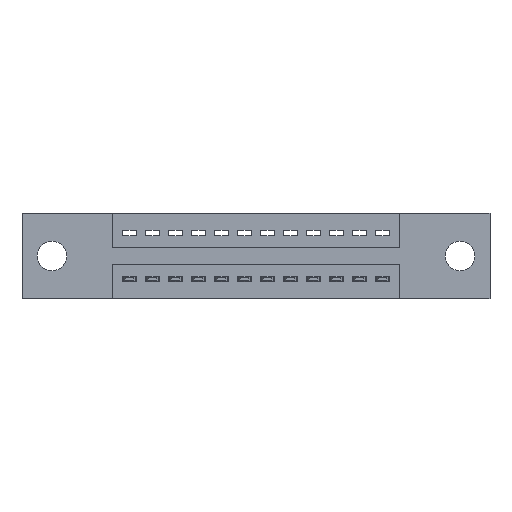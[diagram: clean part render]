
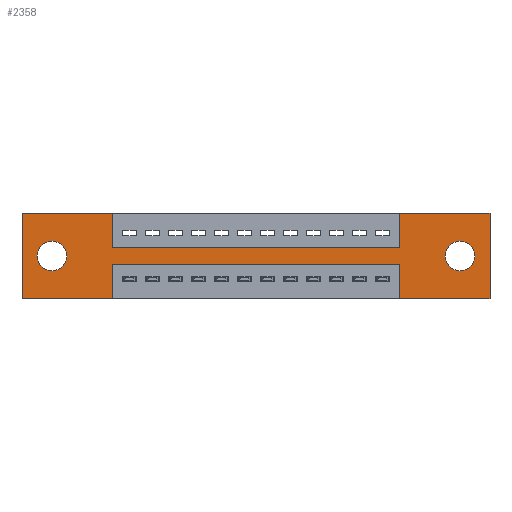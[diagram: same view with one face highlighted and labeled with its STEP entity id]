
A CAD part, front view. The second image highlights one B-rep face of the part: STEP entity #2358.
In plain terms, the highlighted planar face has unit normal (0, -1, 0).
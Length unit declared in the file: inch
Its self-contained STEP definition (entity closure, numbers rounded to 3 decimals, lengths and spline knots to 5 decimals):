
#106 = VECTOR ( 'NONE', #5820, 39.37008 ) ;
#159 = CARTESIAN_POINT ( 'NONE',  ( 2.035, 0., 0. ) ) ;
#206 = LINE ( 'NONE', #3514, #5138 ) ;
#230 = CIRCLE ( 'NONE', #300, 0.064 ) ;
#300 = AXIS2_PLACEMENT_3D ( 'NONE', #12722, #7587, #6706 ) ;
#420 = VERTEX_POINT ( 'NONE', #12027 ) ;
#423 = LINE ( 'NONE', #4810, #106 ) ;
#499 = EDGE_CURVE ( 'NONE', #1969, #12768, #10597, .T. ) ;
#566 = LINE ( 'NONE', #1844, #1185 ) ;
#683 = EDGE_CURVE ( 'NONE', #12281, #10025, #2646, .T. ) ;
#874 = CARTESIAN_POINT ( 'NONE',  ( 0., 0., 0. ) ) ;
#915 = EDGE_LOOP ( 'NONE', ( #11493, #12280, #1550, #6543, #5433, #10860, #11381, #11268, #9116, #10069, #10234, #10438 ) ) ;
#1167 = DIRECTION ( 'NONE',  ( 0., 0., 1. ) ) ;
#1185 = VECTOR ( 'NONE', #2831, 39.37008 ) ;
#1343 = AXIS2_PLACEMENT_3D ( 'NONE', #11222, #5235, #12247 ) ;
#1377 = EDGE_CURVE ( 'NONE', #10025, #3763, #12811, .T. ) ;
#1464 = EDGE_CURVE ( 'NONE', #9595, #420, #11556, .T. ) ;
#1539 = DIRECTION ( 'NONE',  ( 1., 0., 0. ) ) ;
#1550 = ORIENTED_EDGE ( 'NONE', *, *, #7422, .F. ) ;
#1815 = CARTESIAN_POINT ( 'NONE',  ( 1.6425, 0., -0.22 ) ) ;
#1825 = LINE ( 'NONE', #11858, #12153 ) ;
#1844 = CARTESIAN_POINT ( 'NONE',  ( 0., 0., -0.37 ) ) ;
#1969 = VERTEX_POINT ( 'NONE', #10654 ) ;
#2114 = DIRECTION ( 'NONE',  ( 0., 0., -1. ) ) ;
#2358 = ADVANCED_FACE ( 'NONE', ( #2457, #12483, #8075 ), #7083, .T. ) ;
#2457 = FACE_BOUND ( 'NONE', #12046, .T. ) ;
#2481 = VECTOR ( 'NONE', #8828, 39.37008 ) ;
#2585 = CARTESIAN_POINT ( 'NONE',  ( 1.905, 0., -0.249 ) ) ;
#2646 = LINE ( 'NONE', #6172, #8100 ) ;
#2786 = VECTOR ( 'NONE', #1167, 39.37008 ) ;
#2831 = DIRECTION ( 'NONE',  ( -1., 0., 0. ) ) ;
#2841 = DIRECTION ( 'NONE',  ( 0., 0., -1. ) ) ;
#2874 = CARTESIAN_POINT ( 'NONE',  ( 0.3925, 0., -0.22 ) ) ;
#2958 = CARTESIAN_POINT ( 'NONE',  ( 0.3925, 0., 0. ) ) ;
#2996 = CIRCLE ( 'NONE', #1343, 0.064 ) ;
#3005 = EDGE_CURVE ( 'NONE', #10457, #7427, #6411, .T. ) ;
#3021 = LINE ( 'NONE', #2958, #5501 ) ;
#3087 = DIRECTION ( 'NONE',  ( 0., 1., 0. ) ) ;
#3472 = CIRCLE ( 'NONE', #10406, 0.064 ) ;
#3514 = CARTESIAN_POINT ( 'NONE',  ( 0., 0., 0. ) ) ;
#3698 = CARTESIAN_POINT ( 'NONE',  ( 2.035, 0., -0.37 ) ) ;
#3758 = EDGE_CURVE ( 'NONE', #5902, #7552, #230, .T. ) ;
#3763 = VERTEX_POINT ( 'NONE', #9587 ) ;
#4264 = EDGE_CURVE ( 'NONE', #420, #7570, #206, .T. ) ;
#4327 = ORIENTED_EDGE ( 'NONE', *, *, #9861, .T. ) ;
#4484 = DIRECTION ( 'NONE',  ( 0., 0., -1. ) ) ;
#4640 = CARTESIAN_POINT ( 'NONE',  ( 1.6425, 0., -0.15 ) ) ;
#4796 = ORIENTED_EDGE ( 'NONE', *, *, #3758, .T. ) ;
#4810 = CARTESIAN_POINT ( 'NONE',  ( 1.6425, 0., -0.37 ) ) ;
#4867 = DIRECTION ( 'NONE',  ( 1., 0., 0. ) ) ;
#5110 = VERTEX_POINT ( 'NONE', #1815 ) ;
#5138 = VECTOR ( 'NONE', #1539, 39.37008 ) ;
#5165 = EDGE_CURVE ( 'NONE', #9723, #7719, #11215, .T. ) ;
#5235 = DIRECTION ( 'NONE',  ( 0., 1., 0. ) ) ;
#5433 = ORIENTED_EDGE ( 'NONE', *, *, #5165, .F. ) ;
#5501 = VECTOR ( 'NONE', #11880, 39.37008 ) ;
#5617 = CARTESIAN_POINT ( 'NONE',  ( 0.3925, 0., -0.15 ) ) ;
#5638 = CARTESIAN_POINT ( 'NONE',  ( 1.905, 0., -0.185 ) ) ;
#5820 = DIRECTION ( 'NONE',  ( 0., 0., 1. ) ) ;
#5902 = VERTEX_POINT ( 'NONE', #2585 ) ;
#6036 = EDGE_CURVE ( 'NONE', #12768, #9595, #1825, .T. ) ;
#6172 = CARTESIAN_POINT ( 'NONE',  ( 0.3925, 0., -0.15 ) ) ;
#6252 = VECTOR ( 'NONE', #8904, 39.37008 ) ;
#6411 = CIRCLE ( 'NONE', #9010, 0.064 ) ;
#6543 = ORIENTED_EDGE ( 'NONE', *, *, #8403, .F. ) ;
#6706 = DIRECTION ( 'NONE',  ( 0., 0., -1. ) ) ;
#6718 = DIRECTION ( 'NONE',  ( -1., 0., 0. ) ) ;
#6994 = DIRECTION ( 'NONE',  ( 0., -1., 0. ) ) ;
#7083 = PLANE ( 'NONE',  #7494 ) ;
#7099 = CARTESIAN_POINT ( 'NONE',  ( 1.6425, 0., 0. ) ) ;
#7410 = CARTESIAN_POINT ( 'NONE',  ( 1.905, 0., -0.121 ) ) ;
#7422 = EDGE_CURVE ( 'NONE', #10544, #5110, #423, .T. ) ;
#7427 = VERTEX_POINT ( 'NONE', #10896 ) ;
#7494 = AXIS2_PLACEMENT_3D ( 'NONE', #8039, #6994, #2114 ) ;
#7552 = VERTEX_POINT ( 'NONE', #7410 ) ;
#7570 = VERTEX_POINT ( 'NONE', #12541 ) ;
#7587 = DIRECTION ( 'NONE',  ( 0., 1., 0. ) ) ;
#7673 = CARTESIAN_POINT ( 'NONE',  ( 2.035, 0., 0. ) ) ;
#7719 = VERTEX_POINT ( 'NONE', #3698 ) ;
#7902 = CARTESIAN_POINT ( 'NONE',  ( 1.6425, 0., -0.37 ) ) ;
#7999 = LINE ( 'NONE', #874, #9094 ) ;
#8039 = CARTESIAN_POINT ( 'NONE',  ( 0., 0., -0.37 ) ) ;
#8075 = FACE_OUTER_BOUND ( 'NONE', #915, .T. ) ;
#8100 = VECTOR ( 'NONE', #12319, 39.37008 ) ;
#8183 = CARTESIAN_POINT ( 'NONE',  ( 0.13, 0., -0.185 ) ) ;
#8350 = ORIENTED_EDGE ( 'NONE', *, *, #3005, .T. ) ;
#8403 = EDGE_CURVE ( 'NONE', #7719, #10544, #566, .T. ) ;
#8828 = DIRECTION ( 'NONE',  ( 0., 0., 1. ) ) ;
#8894 = VECTOR ( 'NONE', #9421, 39.37008 ) ;
#8904 = DIRECTION ( 'NONE',  ( -1., 0., 0. ) ) ;
#9010 = AXIS2_PLACEMENT_3D ( 'NONE', #8183, #3087, #9149 ) ;
#9094 = VECTOR ( 'NONE', #4867, 39.37008 ) ;
#9116 = ORIENTED_EDGE ( 'NONE', *, *, #9348, .F. ) ;
#9119 = ORIENTED_EDGE ( 'NONE', *, *, #9516, .T. ) ;
#9149 = DIRECTION ( 'NONE',  ( 0., 0., 1. ) ) ;
#9348 = EDGE_CURVE ( 'NONE', #7570, #12281, #3021, .T. ) ;
#9421 = DIRECTION ( 'NONE',  ( 0., 0., -1. ) ) ;
#9446 = DIRECTION ( 'NONE',  ( 0., 1., 0. ) ) ;
#9516 = EDGE_CURVE ( 'NONE', #7552, #5902, #3472, .T. ) ;
#9587 = CARTESIAN_POINT ( 'NONE',  ( 1.6425, 0., 0. ) ) ;
#9595 = VERTEX_POINT ( 'NONE', #12704 ) ;
#9668 = EDGE_CURVE ( 'NONE', #3763, #9723, #7999, .T. ) ;
#9723 = VERTEX_POINT ( 'NONE', #159 ) ;
#9799 = VECTOR ( 'NONE', #2841, 39.37008 ) ;
#9861 = EDGE_CURVE ( 'NONE', #7427, #10457, #2996, .T. ) ;
#10025 = VERTEX_POINT ( 'NONE', #4640 ) ;
#10069 = ORIENTED_EDGE ( 'NONE', *, *, #4264, .F. ) ;
#10192 = EDGE_CURVE ( 'NONE', #5110, #1969, #12231, .T. ) ;
#10233 = EDGE_LOOP ( 'NONE', ( #8350, #4327 ) ) ;
#10234 = ORIENTED_EDGE ( 'NONE', *, *, #1464, .F. ) ;
#10406 = AXIS2_PLACEMENT_3D ( 'NONE', #5638, #9446, #4484 ) ;
#10438 = ORIENTED_EDGE ( 'NONE', *, *, #6036, .F. ) ;
#10448 = CARTESIAN_POINT ( 'NONE',  ( 0.3925, 0., -0.37 ) ) ;
#10457 = VERTEX_POINT ( 'NONE', #11909 ) ;
#10544 = VERTEX_POINT ( 'NONE', #7902 ) ;
#10597 = LINE ( 'NONE', #12377, #8894 ) ;
#10654 = CARTESIAN_POINT ( 'NONE',  ( 0.3925, 0., -0.22 ) ) ;
#10860 = ORIENTED_EDGE ( 'NONE', *, *, #9668, .F. ) ;
#10896 = CARTESIAN_POINT ( 'NONE',  ( 0.13, 0., -0.249 ) ) ;
#11215 = LINE ( 'NONE', #7673, #9799 ) ;
#11222 = CARTESIAN_POINT ( 'NONE',  ( 0.13, 0., -0.185 ) ) ;
#11268 = ORIENTED_EDGE ( 'NONE', *, *, #683, .F. ) ;
#11381 = ORIENTED_EDGE ( 'NONE', *, *, #1377, .F. ) ;
#11493 = ORIENTED_EDGE ( 'NONE', *, *, #499, .F. ) ;
#11556 = LINE ( 'NONE', #12831, #2481 ) ;
#11858 = CARTESIAN_POINT ( 'NONE',  ( 0., 0., -0.37 ) ) ;
#11880 = DIRECTION ( 'NONE',  ( 0., 0., -1. ) ) ;
#11909 = CARTESIAN_POINT ( 'NONE',  ( 0.13, 0., -0.121 ) ) ;
#12027 = CARTESIAN_POINT ( 'NONE',  ( 0., 0., 0. ) ) ;
#12046 = EDGE_LOOP ( 'NONE', ( #9119, #4796 ) ) ;
#12153 = VECTOR ( 'NONE', #6718, 39.37008 ) ;
#12231 = LINE ( 'NONE', #2874, #6252 ) ;
#12247 = DIRECTION ( 'NONE',  ( 0., 0., 1. ) ) ;
#12280 = ORIENTED_EDGE ( 'NONE', *, *, #10192, .F. ) ;
#12281 = VERTEX_POINT ( 'NONE', #5617 ) ;
#12319 = DIRECTION ( 'NONE',  ( 1., 0., 0. ) ) ;
#12377 = CARTESIAN_POINT ( 'NONE',  ( 0.3925, 0., -0.37 ) ) ;
#12483 = FACE_BOUND ( 'NONE', #10233, .T. ) ;
#12541 = CARTESIAN_POINT ( 'NONE',  ( 0.3925, 0., 0. ) ) ;
#12704 = CARTESIAN_POINT ( 'NONE',  ( 0., 0., -0.37 ) ) ;
#12722 = CARTESIAN_POINT ( 'NONE',  ( 1.905, 0., -0.185 ) ) ;
#12768 = VERTEX_POINT ( 'NONE', #10448 ) ;
#12811 = LINE ( 'NONE', #7099, #2786 ) ;
#12831 = CARTESIAN_POINT ( 'NONE',  ( 0., 0., 0. ) ) ;
